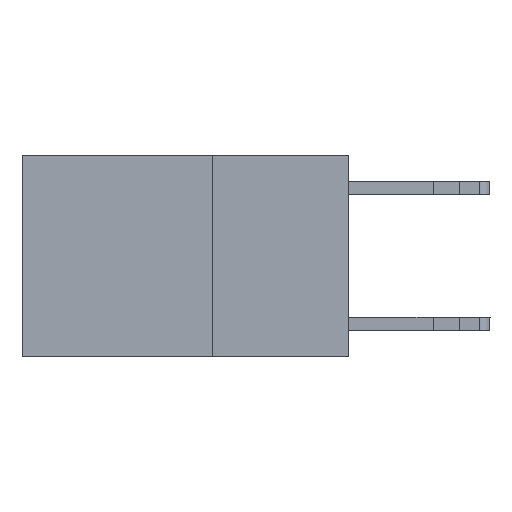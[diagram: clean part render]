
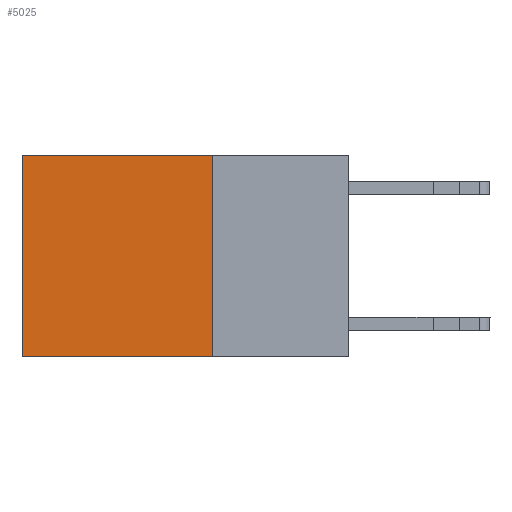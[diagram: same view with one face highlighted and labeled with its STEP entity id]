
A CAD part, left-side view. The second image highlights one B-rep face of the part: STEP entity #5025.
In plain terms, the highlighted planar face has unit normal (-1, 0, 0).
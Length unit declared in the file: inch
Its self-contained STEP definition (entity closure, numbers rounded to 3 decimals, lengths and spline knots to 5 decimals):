
#124 = LINE ( 'NONE', #3063, #1220 ) ;
#353 = VERTEX_POINT ( 'NONE', #16140 ) ;
#1175 = LINE ( 'NONE', #10474, #17804 ) ;
#1220 = VECTOR ( 'NONE', #16225, 39.37008 ) ;
#1689 = DIRECTION ( 'NONE',  ( 1., 0., 0. ) ) ;
#3063 = CARTESIAN_POINT ( 'NONE',  ( 0.2625, 0.25, 0. ) ) ;
#3291 = EDGE_CURVE ( 'NONE', #17190, #353, #3893, .T. ) ;
#3770 = CARTESIAN_POINT ( 'NONE',  ( 0.2625, 0.6, 0. ) ) ;
#3893 = LINE ( 'NONE', #15567, #16073 ) ;
#3973 = VECTOR ( 'NONE', #5209, 39.37008 ) ;
#4835 = DIRECTION ( 'NONE',  ( 0., 0., -1. ) ) ;
#4938 = VERTEX_POINT ( 'NONE', #5738 ) ;
#5025 = ADVANCED_FACE ( 'NONE', ( #16818 ), #16715, .F. ) ;
#5209 = DIRECTION ( 'NONE',  ( 0., 0., -1. ) ) ;
#5307 = LINE ( 'NONE', #6512, #3973 ) ;
#5738 = CARTESIAN_POINT ( 'NONE',  ( 0.2625, 0.6, -0.37 ) ) ;
#6044 = CARTESIAN_POINT ( 'NONE',  ( 0.2625, 0.25, 0. ) ) ;
#6445 = ORIENTED_EDGE ( 'NONE', *, *, #12269, .F. ) ;
#6512 = CARTESIAN_POINT ( 'NONE',  ( 0.2625, 0.6, 0. ) ) ;
#7356 = ORIENTED_EDGE ( 'NONE', *, *, #3291, .F. ) ;
#8004 = ORIENTED_EDGE ( 'NONE', *, *, #14842, .T. ) ;
#8622 = ORIENTED_EDGE ( 'NONE', *, *, #11747, .T. ) ;
#9455 = CARTESIAN_POINT ( 'NONE',  ( 0.2625, 0.25, 0. ) ) ;
#10474 = CARTESIAN_POINT ( 'NONE',  ( 0.2625, 0.25, -0.37 ) ) ;
#11199 = AXIS2_PLACEMENT_3D ( 'NONE', #6044, #1689, #4835 ) ;
#11589 = VERTEX_POINT ( 'NONE', #3770 ) ;
#11747 = EDGE_CURVE ( 'NONE', #17190, #11589, #124, .T. ) ;
#12269 = EDGE_CURVE ( 'NONE', #353, #4938, #1175, .T. ) ;
#13501 = EDGE_LOOP ( 'NONE', ( #8004, #6445, #7356, #8622 ) ) ;
#13548 = DIRECTION ( 'NONE',  ( 0., 1., 0. ) ) ;
#14002 = DIRECTION ( 'NONE',  ( 0., 0., -1. ) ) ;
#14842 = EDGE_CURVE ( 'NONE', #11589, #4938, #5307, .T. ) ;
#15567 = CARTESIAN_POINT ( 'NONE',  ( 0.2625, 0.25, 0. ) ) ;
#16073 = VECTOR ( 'NONE', #14002, 39.37008 ) ;
#16140 = CARTESIAN_POINT ( 'NONE',  ( 0.2625, 0.25, -0.37 ) ) ;
#16225 = DIRECTION ( 'NONE',  ( 0., 1., 0. ) ) ;
#16715 = PLANE ( 'NONE',  #11199 ) ;
#16818 = FACE_OUTER_BOUND ( 'NONE', #13501, .T. ) ;
#17190 = VERTEX_POINT ( 'NONE', #9455 ) ;
#17804 = VECTOR ( 'NONE', #13548, 39.37008 ) ;
